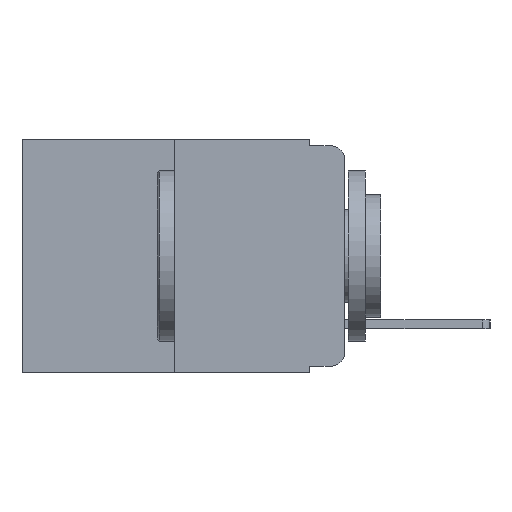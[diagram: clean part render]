
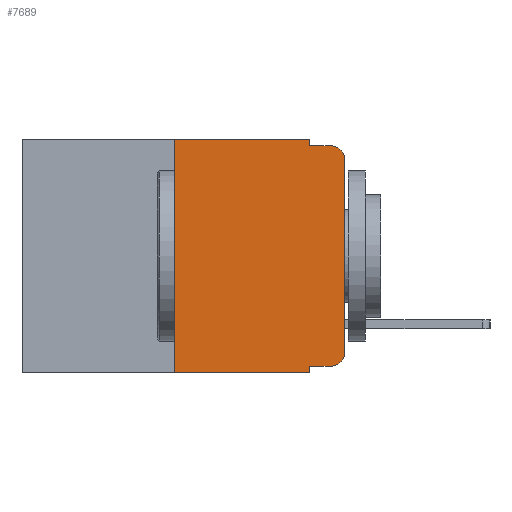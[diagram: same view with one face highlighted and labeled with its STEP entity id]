
A CAD part, left-side view. The second image highlights one B-rep face of the part: STEP entity #7689.
In plain terms, the highlighted planar face has unit normal (-1, 0, 0).
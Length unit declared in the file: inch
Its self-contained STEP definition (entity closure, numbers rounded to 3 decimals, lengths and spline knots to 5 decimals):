
#16 = EDGE_CURVE ( 'NONE', #18652, #21829, #17949, .T. ) ;
#66 = EDGE_CURVE ( 'NONE', #21829, #2418, #9283, .T. ) ;
#97 = EDGE_CURVE ( 'NONE', #17480, #2418, #6841, .T. ) ;
#101 = EDGE_CURVE ( 'NONE', #18459, #17480, #20773, .T. ) ;
#145 = EDGE_CURVE ( 'NONE', #8505, #3773, #18711, .T. ) ;
#148 = EDGE_CURVE ( 'NONE', #14933, #15398, #22583, .T. ) ;
#182 = EDGE_CURVE ( 'NONE', #14933, #15532, #8400, .T. ) ;
#185 = EDGE_CURVE ( 'NONE', #15532, #18652, #17681, .T. ) ;
#1280 = VECTOR ( 'NONE', #17226, 39.37008 ) ;
#1695 = ORIENTED_EDGE ( 'NONE', *, *, #66, .T. ) ;
#2418 = VERTEX_POINT ( 'NONE', #21155 ) ;
#2524 = VECTOR ( 'NONE', #22959, 39.37008 ) ;
#2742 = DIRECTION ( 'NONE',  ( 0., 0., -1. ) ) ;
#3019 = DIRECTION ( 'NONE',  ( -1., 0., 0. ) ) ;
#3773 = VERTEX_POINT ( 'NONE', #20601 ) ;
#5866 = EDGE_CURVE ( 'NONE', #8505, #15398, #18876, .T. ) ;
#6824 = PLANE ( 'NONE',  #20276 ) ;
#6841 = LINE ( 'NONE', #19127, #1280 ) ;
#7689 = ADVANCED_FACE ( 'NONE', ( #9944 ), #6824, .F. ) ;
#8400 = LINE ( 'NONE', #8949, #14175 ) ;
#8485 = CARTESIAN_POINT ( 'NONE',  ( 0., 0., 0. ) ) ;
#8505 = VERTEX_POINT ( 'NONE', #11036 ) ;
#8512 = DIRECTION ( 'NONE',  ( -1., 0., 0. ) ) ;
#8614 = LINE ( 'NONE', #21294, #2524 ) ;
#8949 = CARTESIAN_POINT ( 'NONE',  ( 0., 0.051, -0.333 ) ) ;
#8965 = CARTESIAN_POINT ( 'NONE',  ( 0., 0.051, 0. ) ) ;
#9091 = CARTESIAN_POINT ( 'NONE',  ( 0., 0.02, -0.333 ) ) ;
#9283 = CIRCLE ( 'NONE', #11473, 0.02 ) ;
#9575 = VECTOR ( 'NONE', #10774, 39.37008 ) ;
#9944 = FACE_OUTER_BOUND ( 'NONE', #16085, .T. ) ;
#9945 = ORIENTED_EDGE ( 'NONE', *, *, #148, .F. ) ;
#10223 = ORIENTED_EDGE ( 'NONE', *, *, #21907, .F. ) ;
#10774 = DIRECTION ( 'NONE',  ( 0., 0., 1. ) ) ;
#11036 = CARTESIAN_POINT ( 'NONE',  ( 0., 0.25, -0.343 ) ) ;
#11473 = AXIS2_PLACEMENT_3D ( 'NONE', #11729, #8512, #16977 ) ;
#11729 = CARTESIAN_POINT ( 'NONE',  ( 0., 0.02, -0.03 ) ) ;
#11837 = VECTOR ( 'NONE', #17326, 39.37008 ) ;
#12457 = DIRECTION ( 'NONE',  ( 0., 0., -1. ) ) ;
#13316 = CARTESIAN_POINT ( 'NONE',  ( 0., 0.051, -0.333 ) ) ;
#13398 = VECTOR ( 'NONE', #16655, 39.37008 ) ;
#13820 = VECTOR ( 'NONE', #22279, 39.37008 ) ;
#14033 = CARTESIAN_POINT ( 'NONE',  ( 0., 0.473, 0. ) ) ;
#14036 = CARTESIAN_POINT ( 'NONE',  ( 0., 0.051, -0.01 ) ) ;
#14083 = CARTESIAN_POINT ( 'NONE',  ( 0., 0.25, 0. ) ) ;
#14175 = VECTOR ( 'NONE', #22636, 39.37008 ) ;
#14769 = ORIENTED_EDGE ( 'NONE', *, *, #145, .F. ) ;
#14813 = DIRECTION ( 'NONE',  ( 0., 0., -1. ) ) ;
#14933 = VERTEX_POINT ( 'NONE', #13316 ) ;
#15028 = ORIENTED_EDGE ( 'NONE', *, *, #16, .T. ) ;
#15398 = VERTEX_POINT ( 'NONE', #20813 ) ;
#15401 = CARTESIAN_POINT ( 'NONE',  ( 0., 0.051, 0. ) ) ;
#15532 = VERTEX_POINT ( 'NONE', #9091 ) ;
#15598 = ORIENTED_EDGE ( 'NONE', *, *, #182, .T. ) ;
#16085 = EDGE_LOOP ( 'NONE', ( #15028, #1695, #17207, #21598, #10223, #14769, #16943, #9945, #15598, #21621 ) ) ;
#16182 = CARTESIAN_POINT ( 'NONE',  ( 0., 0., -0.313 ) ) ;
#16655 = DIRECTION ( 'NONE',  ( 0., 0., 1. ) ) ;
#16943 = ORIENTED_EDGE ( 'NONE', *, *, #5866, .T. ) ;
#16977 = DIRECTION ( 'NONE',  ( 0., 0., -1. ) ) ;
#17207 = ORIENTED_EDGE ( 'NONE', *, *, #97, .F. ) ;
#17226 = DIRECTION ( 'NONE',  ( 0., -1., 0. ) ) ;
#17326 = DIRECTION ( 'NONE',  ( 0., 0., -1. ) ) ;
#17480 = VERTEX_POINT ( 'NONE', #14036 ) ;
#17681 = CIRCLE ( 'NONE', #19394, 0.02 ) ;
#17949 = LINE ( 'NONE', #8485, #13398 ) ;
#18189 = VECTOR ( 'NONE', #14813, 39.37008 ) ;
#18459 = VERTEX_POINT ( 'NONE', #8965 ) ;
#18652 = VERTEX_POINT ( 'NONE', #16182 ) ;
#18711 = LINE ( 'NONE', #14083, #9575 ) ;
#18876 = LINE ( 'NONE', #20632, #13820 ) ;
#19127 = CARTESIAN_POINT ( 'NONE',  ( 0., 0.051, -0.01 ) ) ;
#19394 = AXIS2_PLACEMENT_3D ( 'NONE', #22587, #3019, #2742 ) ;
#20276 = AXIS2_PLACEMENT_3D ( 'NONE', #14033, #22474, #12457 ) ;
#20301 = CARTESIAN_POINT ( 'NONE',  ( 0., 0.051, 0. ) ) ;
#20601 = CARTESIAN_POINT ( 'NONE',  ( 0., 0.25, 0. ) ) ;
#20632 = CARTESIAN_POINT ( 'NONE',  ( 0., 0.473, -0.343 ) ) ;
#20773 = LINE ( 'NONE', #20301, #11837 ) ;
#20813 = CARTESIAN_POINT ( 'NONE',  ( 0., 0.051, -0.343 ) ) ;
#21155 = CARTESIAN_POINT ( 'NONE',  ( 0., 0.02, -0.01 ) ) ;
#21294 = CARTESIAN_POINT ( 'NONE',  ( 0., 0.473, 0. ) ) ;
#21598 = ORIENTED_EDGE ( 'NONE', *, *, #101, .F. ) ;
#21621 = ORIENTED_EDGE ( 'NONE', *, *, #185, .T. ) ;
#21829 = VERTEX_POINT ( 'NONE', #22811 ) ;
#21907 = EDGE_CURVE ( 'NONE', #3773, #18459, #8614, .T. ) ;
#22279 = DIRECTION ( 'NONE',  ( 0., -1., 0. ) ) ;
#22474 = DIRECTION ( 'NONE',  ( 1., 0., 0. ) ) ;
#22583 = LINE ( 'NONE', #15401, #18189 ) ;
#22587 = CARTESIAN_POINT ( 'NONE',  ( 0., 0.02, -0.313 ) ) ;
#22636 = DIRECTION ( 'NONE',  ( 0., -1., 0. ) ) ;
#22811 = CARTESIAN_POINT ( 'NONE',  ( 0., 0., -0.03 ) ) ;
#22959 = DIRECTION ( 'NONE',  ( 0., -1., 0. ) ) ;
